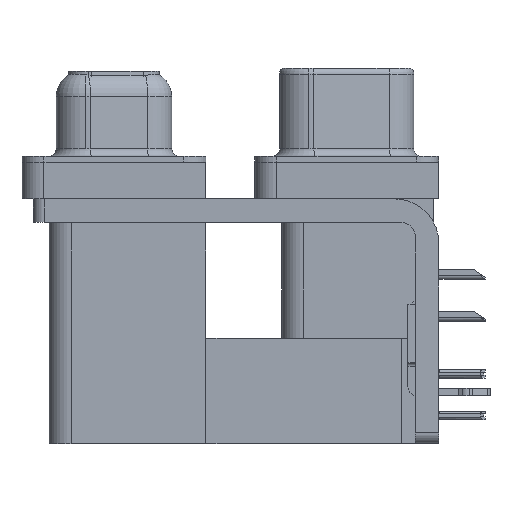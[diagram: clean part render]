
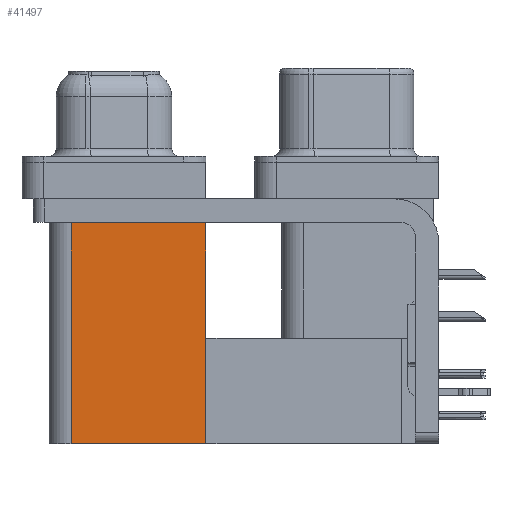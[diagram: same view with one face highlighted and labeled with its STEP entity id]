
A CAD part, left-side view. The second image highlights one B-rep face of the part: STEP entity #41497.
In plain terms, the highlighted planar face has unit normal (-1, 0, 0).
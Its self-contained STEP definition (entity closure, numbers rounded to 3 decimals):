
#344 = CARTESIAN_POINT ( 'NONE',  ( 3.765, 9.6, -19.2 ) ) ;
#564 = DIRECTION ( 'NONE',  ( 1., 0., 0. ) ) ;
#1032 = ORIENTED_EDGE ( 'NONE', *, *, #27520, .F. ) ;
#4270 = VERTEX_POINT ( 'NONE', #36151 ) ;
#5622 = DIRECTION ( 'NONE',  ( 0., 1., 0. ) ) ;
#7211 = CARTESIAN_POINT ( 'NONE',  ( 3.765, 18.8, -19.2 ) ) ;
#7386 = DIRECTION ( 'NONE',  ( 0., 0., -1. ) ) ;
#9731 = DIRECTION ( 'NONE',  ( 0., 0., 1. ) ) ;
#9933 = EDGE_LOOP ( 'NONE', ( #35153, #16241, #1032, #35510 ) ) ;
#11173 = CARTESIAN_POINT ( 'NONE',  ( 3.765, 9.6, -19.2 ) ) ;
#11174 = VERTEX_POINT ( 'NONE', #40680 ) ;
#13058 = AXIS2_PLACEMENT_3D ( 'NONE', #344, #564, #7386 ) ;
#16241 = ORIENTED_EDGE ( 'NONE', *, *, #39143, .F. ) ;
#17290 = PLANE ( 'NONE',  #13058 ) ;
#22918 = CARTESIAN_POINT ( 'NONE',  ( 3.765, 9.6, -2.5 ) ) ;
#24583 = DIRECTION ( 'NONE',  ( 0., 0., 1. ) ) ;
#25081 = VERTEX_POINT ( 'NONE', #7211 ) ;
#26328 = VECTOR ( 'NONE', #9731, 1000. ) ;
#26442 = CARTESIAN_POINT ( 'NONE',  ( 3.765, 18.8, -19.2 ) ) ;
#27167 = FACE_OUTER_BOUND ( 'NONE', #9933, .T. ) ;
#27520 = EDGE_CURVE ( 'NONE', #11174, #25081, #37185, .T. ) ;
#29569 = LINE ( 'NONE', #31985, #39204 ) ;
#30457 = EDGE_CURVE ( 'NONE', #31078, #4270, #29569, .T. ) ;
#30802 = DIRECTION ( 'NONE',  ( 0., 1., 0. ) ) ;
#31078 = VERTEX_POINT ( 'NONE', #22918 ) ;
#31985 = CARTESIAN_POINT ( 'NONE',  ( 3.765, 9.6, -2.5 ) ) ;
#35153 = ORIENTED_EDGE ( 'NONE', *, *, #30457, .T. ) ;
#35510 = ORIENTED_EDGE ( 'NONE', *, *, #43172, .T. ) ;
#36151 = CARTESIAN_POINT ( 'NONE',  ( 3.765, 18.8, -2.5 ) ) ;
#37185 = LINE ( 'NONE', #37612, #38419 ) ;
#37612 = CARTESIAN_POINT ( 'NONE',  ( 3.765, 9.6, -19.2 ) ) ;
#38419 = VECTOR ( 'NONE', #30802, 1000. ) ;
#38434 = VECTOR ( 'NONE', #24583, 1000. ) ;
#39143 = EDGE_CURVE ( 'NONE', #25081, #4270, #39424, .T. ) ;
#39204 = VECTOR ( 'NONE', #5622, 1000. ) ;
#39424 = LINE ( 'NONE', #26442, #26328 ) ;
#40680 = CARTESIAN_POINT ( 'NONE',  ( 3.765, 9.6, -19.2 ) ) ;
#41278 = LINE ( 'NONE', #11173, #38434 ) ;
#41497 = ADVANCED_FACE ( 'NONE', ( #27167 ), #17290, .F. ) ;
#43172 = EDGE_CURVE ( 'NONE', #11174, #31078, #41278, .T. ) ;
